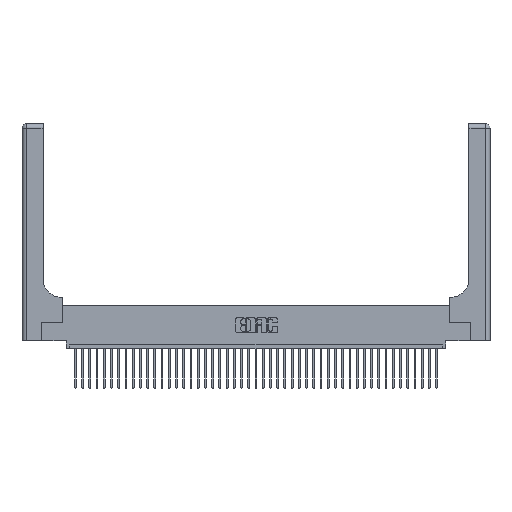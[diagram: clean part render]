
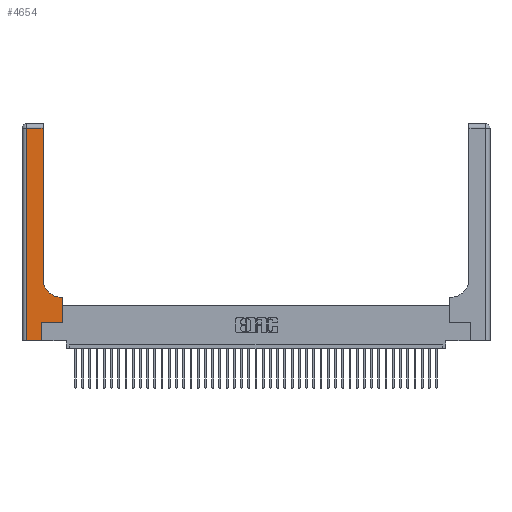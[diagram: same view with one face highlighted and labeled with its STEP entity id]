
A CAD part, top view. The second image highlights one B-rep face of the part: STEP entity #4654.
In plain terms, the highlighted planar face has unit normal (0, 0, 1).
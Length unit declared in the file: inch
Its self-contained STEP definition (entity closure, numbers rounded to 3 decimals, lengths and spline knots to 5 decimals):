
#489 = DIRECTION ( 'NONE',  ( 0., -1., 0. ) ) ;
#715 = LINE ( 'NONE', #35149, #22248 ) ;
#761 = EDGE_CURVE ( 'NONE', #26940, #39619, #36779, .T. ) ;
#920 = CARTESIAN_POINT ( 'NONE',  ( 0.269, 0., 0.37 ) ) ;
#1706 = DIRECTION ( 'NONE',  ( 1., 0., 0. ) ) ;
#2454 = CARTESIAN_POINT ( 'NONE',  ( 0.5585, 0.25, 0.37 ) ) ;
#2547 = VERTEX_POINT ( 'NONE', #7884 ) ;
#2866 = DIRECTION ( 'NONE',  ( 0., 1., 0. ) ) ;
#3155 = ORIENTED_EDGE ( 'NONE', *, *, #23726, .T. ) ;
#3414 = EDGE_CURVE ( 'NONE', #19932, #34127, #17548, .T. ) ;
#4320 = CARTESIAN_POINT ( 'NONE',  ( 0.5585, 0.6, 0.37 ) ) ;
#4654 = ADVANCED_FACE ( 'NONE', ( #7281 ), #18937, .F. ) ;
#5675 = DIRECTION ( 'NONE',  ( 1., 0., 0. ) ) ;
#6388 = VECTOR ( 'NONE', #16776, 39.37008 ) ;
#7281 = FACE_OUTER_BOUND ( 'NONE', #7785, .T. ) ;
#7739 = ORIENTED_EDGE ( 'NONE', *, *, #15882, .T. ) ;
#7785 = EDGE_LOOP ( 'NONE', ( #30068, #11495, #31856, #7739, #3155, #33154, #24306, #27207, #23655 ) ) ;
#7884 = CARTESIAN_POINT ( 'NONE',  ( 0.269, 0.25, 0.37 ) ) ;
#8602 = EDGE_CURVE ( 'NONE', #9525, #26940, #29577, .T. ) ;
#8937 = VECTOR ( 'NONE', #23816, 39.37008 ) ;
#9098 = DIRECTION ( 'NONE',  ( -1., 0., 0. ) ) ;
#9525 = VERTEX_POINT ( 'NONE', #27013 ) ;
#10191 = LINE ( 'NONE', #20855, #11741 ) ;
#11006 = EDGE_CURVE ( 'NONE', #37427, #19932, #40210, .T. ) ;
#11495 = ORIENTED_EDGE ( 'NONE', *, *, #3414, .T. ) ;
#11741 = VECTOR ( 'NONE', #1706, 39.37008 ) ;
#13503 = LINE ( 'NONE', #23643, #6388 ) ;
#14689 = VECTOR ( 'NONE', #20919, 39.37008 ) ;
#15603 = CARTESIAN_POINT ( 'NONE',  ( 0.2915, 0.85, 0.37 ) ) ;
#15882 = EDGE_CURVE ( 'NONE', #26566, #21845, #10191, .T. ) ;
#16062 = DIRECTION ( 'NONE',  ( -1., 0., 0. ) ) ;
#16776 = DIRECTION ( 'NONE',  ( 1., 0., 0. ) ) ;
#16966 = CARTESIAN_POINT ( 'NONE',  ( 0.2915, 2.94, 0.37 ) ) ;
#17128 = EDGE_CURVE ( 'NONE', #39619, #37427, #17245, .T. ) ;
#17245 = CIRCLE ( 'NONE', #39467, 0.25 ) ;
#17548 = LINE ( 'NONE', #35751, #34006 ) ;
#17749 = VECTOR ( 'NONE', #31423, 39.37008 ) ;
#18937 = PLANE ( 'NONE',  #35900 ) ;
#19932 = VERTEX_POINT ( 'NONE', #16966 ) ;
#20097 = CARTESIAN_POINT ( 'NONE',  ( 0.06, 3., 0.37 ) ) ;
#20103 = CARTESIAN_POINT ( 'NONE',  ( 0.5415, 0.6, 0.37 ) ) ;
#20855 = CARTESIAN_POINT ( 'NONE',  ( 0., 0., 0.37 ) ) ;
#20919 = DIRECTION ( 'NONE',  ( -1., 0., 0. ) ) ;
#21845 = VERTEX_POINT ( 'NONE', #920 ) ;
#22248 = VECTOR ( 'NONE', #2866, 39.37008 ) ;
#23541 = EDGE_CURVE ( 'NONE', #34127, #26566, #31556, .T. ) ;
#23643 = CARTESIAN_POINT ( 'NONE',  ( 0.269, 0.25, 0.37 ) ) ;
#23655 = ORIENTED_EDGE ( 'NONE', *, *, #17128, .T. ) ;
#23726 = EDGE_CURVE ( 'NONE', #21845, #2547, #715, .T. ) ;
#23816 = DIRECTION ( 'NONE',  ( 0., 1., 0. ) ) ;
#24306 = ORIENTED_EDGE ( 'NONE', *, *, #8602, .T. ) ;
#26566 = VERTEX_POINT ( 'NONE', #29315 ) ;
#26940 = VERTEX_POINT ( 'NONE', #4320 ) ;
#27013 = CARTESIAN_POINT ( 'NONE',  ( 0.5585, 0.25, 0.37 ) ) ;
#27119 = CARTESIAN_POINT ( 'NONE',  ( 0.2915, 3., 0.37 ) ) ;
#27207 = ORIENTED_EDGE ( 'NONE', *, *, #761, .T. ) ;
#29315 = CARTESIAN_POINT ( 'NONE',  ( 0.06, 0., 0.37 ) ) ;
#29577 = LINE ( 'NONE', #2454, #17749 ) ;
#29743 = CARTESIAN_POINT ( 'NONE',  ( 0.06, 2.94, 0.37 ) ) ;
#30068 = ORIENTED_EDGE ( 'NONE', *, *, #11006, .T. ) ;
#31423 = DIRECTION ( 'NONE',  ( 0., 1., 0. ) ) ;
#31469 = CARTESIAN_POINT ( 'NONE',  ( 0., 3., 0.37 ) ) ;
#31556 = LINE ( 'NONE', #20097, #40783 ) ;
#31856 = ORIENTED_EDGE ( 'NONE', *, *, #23541, .T. ) ;
#33154 = ORIENTED_EDGE ( 'NONE', *, *, #40267, .T. ) ;
#34006 = VECTOR ( 'NONE', #16062, 39.37008 ) ;
#34127 = VERTEX_POINT ( 'NONE', #29743 ) ;
#35149 = CARTESIAN_POINT ( 'NONE',  ( 0.269, 0., 0.37 ) ) ;
#35332 = CARTESIAN_POINT ( 'NONE',  ( 0.5415, 0.85, 0.37 ) ) ;
#35751 = CARTESIAN_POINT ( 'NONE',  ( 0., 2.94, 0.37 ) ) ;
#35900 = AXIS2_PLACEMENT_3D ( 'NONE', #31469, #41775, #9098 ) ;
#36779 = LINE ( 'NONE', #39915, #14689 ) ;
#37427 = VERTEX_POINT ( 'NONE', #15603 ) ;
#39467 = AXIS2_PLACEMENT_3D ( 'NONE', #35332, #41625, #5675 ) ;
#39619 = VERTEX_POINT ( 'NONE', #20103 ) ;
#39915 = CARTESIAN_POINT ( 'NONE',  ( 0.2915, 0.6, 0.37 ) ) ;
#40210 = LINE ( 'NONE', #27119, #8937 ) ;
#40267 = EDGE_CURVE ( 'NONE', #2547, #9525, #13503, .T. ) ;
#40783 = VECTOR ( 'NONE', #489, 39.37008 ) ;
#41625 = DIRECTION ( 'NONE',  ( 0., 0., -1. ) ) ;
#41775 = DIRECTION ( 'NONE',  ( 0., 0., -1. ) ) ;
